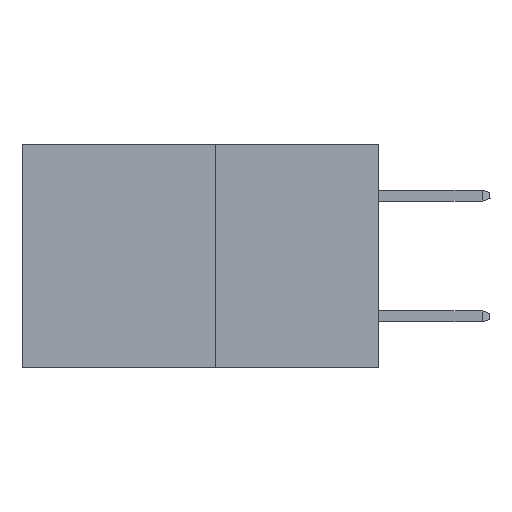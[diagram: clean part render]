
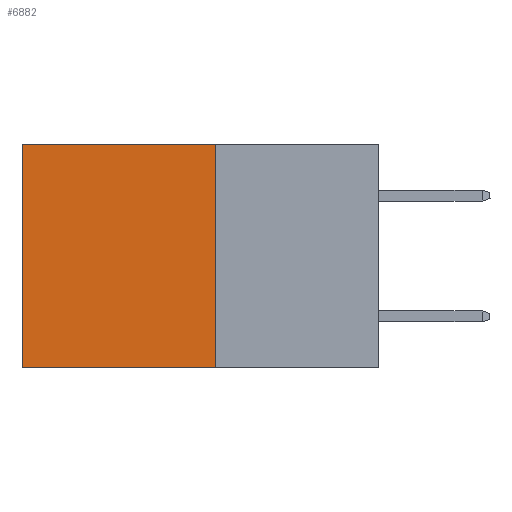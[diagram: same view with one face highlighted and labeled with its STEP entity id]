
A CAD part, left-side view. The second image highlights one B-rep face of the part: STEP entity #6882.
In plain terms, the highlighted planar face has unit normal (-1, 0, 0).
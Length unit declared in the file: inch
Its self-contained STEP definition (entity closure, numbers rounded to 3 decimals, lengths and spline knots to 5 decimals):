
#519 = ORIENTED_EDGE ( 'NONE', *, *, #10719, .T. ) ;
#898 = PLANE ( 'NONE',  #8770 ) ;
#906 = CARTESIAN_POINT ( 'NONE',  ( 0.277, 0.27, 0. ) ) ;
#1015 = VECTOR ( 'NONE', #8740, 39.37008 ) ;
#1067 = DIRECTION ( 'NONE',  ( 0., 1., 0. ) ) ;
#1337 = LINE ( 'NONE', #10207, #6591 ) ;
#1632 = ORIENTED_EDGE ( 'NONE', *, *, #7448, .F. ) ;
#1780 = DIRECTION ( 'NONE',  ( 0., 0., -1. ) ) ;
#2589 = CARTESIAN_POINT ( 'NONE',  ( 0.277, 0.27, 0. ) ) ;
#2740 = EDGE_CURVE ( 'NONE', #10298, #11157, #3408, .T. ) ;
#2866 = EDGE_LOOP ( 'NONE', ( #519, #6171, #1632, #7967 ) ) ;
#3096 = VERTEX_POINT ( 'NONE', #3303 ) ;
#3303 = CARTESIAN_POINT ( 'NONE',  ( 0.277, 0.59, -0.37 ) ) ;
#3408 = LINE ( 'NONE', #906, #10120 ) ;
#3685 = VERTEX_POINT ( 'NONE', #11063 ) ;
#4063 = CARTESIAN_POINT ( 'NONE',  ( 0.277, 0.27, -0.37 ) ) ;
#4508 = EDGE_CURVE ( 'NONE', #3685, #3096, #5924, .T. ) ;
#4806 = DIRECTION ( 'NONE',  ( 0., 0., -1. ) ) ;
#5261 = FACE_OUTER_BOUND ( 'NONE', #2866, .T. ) ;
#5480 = CARTESIAN_POINT ( 'NONE',  ( 0.277, 0.59, 0. ) ) ;
#5771 = CARTESIAN_POINT ( 'NONE',  ( 0.277, 0.59, -0.37 ) ) ;
#5924 = LINE ( 'NONE', #4063, #1015 ) ;
#6171 = ORIENTED_EDGE ( 'NONE', *, *, #4508, .F. ) ;
#6591 = VECTOR ( 'NONE', #4806, 39.37008 ) ;
#6882 = ADVANCED_FACE ( 'NONE', ( #5261 ), #898, .F. ) ;
#7347 = DIRECTION ( 'NONE',  ( 1., 0., 0. ) ) ;
#7448 = EDGE_CURVE ( 'NONE', #10298, #3685, #1337, .T. ) ;
#7967 = ORIENTED_EDGE ( 'NONE', *, *, #2740, .T. ) ;
#8740 = DIRECTION ( 'NONE',  ( 0., 1., 0. ) ) ;
#8770 = AXIS2_PLACEMENT_3D ( 'NONE', #10755, #7347, #1780 ) ;
#9036 = VECTOR ( 'NONE', #10238, 39.37008 ) ;
#10120 = VECTOR ( 'NONE', #1067, 39.37008 ) ;
#10207 = CARTESIAN_POINT ( 'NONE',  ( 0.277, 0.27, -0.37 ) ) ;
#10238 = DIRECTION ( 'NONE',  ( 0., 0., -1. ) ) ;
#10298 = VERTEX_POINT ( 'NONE', #2589 ) ;
#10719 = EDGE_CURVE ( 'NONE', #11157, #3096, #11300, .T. ) ;
#10755 = CARTESIAN_POINT ( 'NONE',  ( 0.277, 0.27, -0.37 ) ) ;
#11063 = CARTESIAN_POINT ( 'NONE',  ( 0.277, 0.27, -0.37 ) ) ;
#11157 = VERTEX_POINT ( 'NONE', #5480 ) ;
#11300 = LINE ( 'NONE', #5771, #9036 ) ;
